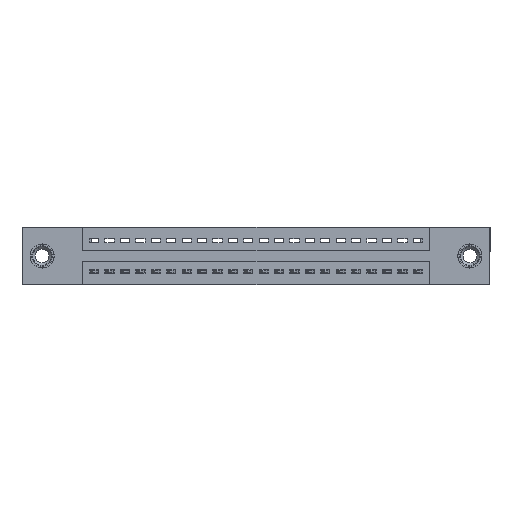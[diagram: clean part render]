
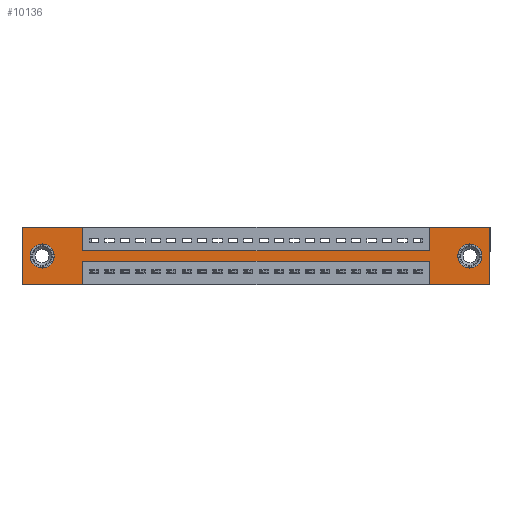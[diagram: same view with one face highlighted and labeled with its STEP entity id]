
A CAD part, front view. The second image highlights one B-rep face of the part: STEP entity #10136.
In plain terms, the highlighted planar face has unit normal (0, -1, 0).
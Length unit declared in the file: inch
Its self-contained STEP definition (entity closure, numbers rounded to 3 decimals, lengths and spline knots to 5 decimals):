
#239 = CARTESIAN_POINT ( 'NONE',  ( 3.035, 0., 0. ) ) ;
#268 = VERTEX_POINT ( 'NONE', #17367 ) ;
#348 = CARTESIAN_POINT ( 'NONE',  ( 2.905, 0., -0.107 ) ) ;
#859 = ORIENTED_EDGE ( 'NONE', *, *, #13881, .T. ) ;
#918 = LINE ( 'NONE', #5117, #19272 ) ;
#1190 = ORIENTED_EDGE ( 'NONE', *, *, #11688, .T. ) ;
#1259 = CARTESIAN_POINT ( 'NONE',  ( 3.035, 0., -0.37 ) ) ;
#1475 = VECTOR ( 'NONE', #5747, 39.37008 ) ;
#1801 = FACE_BOUND ( 'NONE', #2413, .T. ) ;
#2102 = VECTOR ( 'NONE', #16016, 39.37008 ) ;
#2111 = CARTESIAN_POINT ( 'NONE',  ( 0.13, 0., -0.185 ) ) ;
#2248 = EDGE_LOOP ( 'NONE', ( #1190, #8141 ) ) ;
#2413 = EDGE_LOOP ( 'NONE', ( #859, #3671 ) ) ;
#2635 = PLANE ( 'NONE',  #16412 ) ;
#2833 = LINE ( 'NONE', #17756, #11356 ) ;
#3108 = CARTESIAN_POINT ( 'NONE',  ( 2.6425, 0., -0.22 ) ) ;
#3216 = CARTESIAN_POINT ( 'NONE',  ( 2.6425, 0., -0.37 ) ) ;
#3261 = CARTESIAN_POINT ( 'NONE',  ( 0., 0., -0.37 ) ) ;
#3460 = CARTESIAN_POINT ( 'NONE',  ( 0.3925, 0., -0.37 ) ) ;
#3671 = ORIENTED_EDGE ( 'NONE', *, *, #16153, .T. ) ;
#3738 = VECTOR ( 'NONE', #13665, 39.37008 ) ;
#3745 = VERTEX_POINT ( 'NONE', #17710 ) ;
#3965 = EDGE_CURVE ( 'NONE', #14811, #12699, #20220, .T. ) ;
#4048 = CIRCLE ( 'NONE', #10600, 0.078 ) ;
#4083 = CARTESIAN_POINT ( 'NONE',  ( 0., 0., -0.37 ) ) ;
#4700 = DIRECTION ( 'NONE',  ( 0., 0., -1. ) ) ;
#4835 = ORIENTED_EDGE ( 'NONE', *, *, #10574, .F. ) ;
#5117 = CARTESIAN_POINT ( 'NONE',  ( 0., 0., 0. ) ) ;
#5172 = FACE_OUTER_BOUND ( 'NONE', #19229, .T. ) ;
#5348 = ORIENTED_EDGE ( 'NONE', *, *, #20519, .F. ) ;
#5518 = EDGE_CURVE ( 'NONE', #268, #15075, #14728, .T. ) ;
#5523 = AXIS2_PLACEMENT_3D ( 'NONE', #21179, #11009, #7885 ) ;
#5589 = DIRECTION ( 'NONE',  ( 0., 0., 1. ) ) ;
#5600 = CARTESIAN_POINT ( 'NONE',  ( 2.905, 0., -0.263 ) ) ;
#5620 = EDGE_CURVE ( 'NONE', #21409, #8973, #2833, .T. ) ;
#5747 = DIRECTION ( 'NONE',  ( 0., 0., -1. ) ) ;
#5774 = VERTEX_POINT ( 'NONE', #9091 ) ;
#5919 = FACE_BOUND ( 'NONE', #2248, .T. ) ;
#5966 = VECTOR ( 'NONE', #13341, 39.37008 ) ;
#6028 = VERTEX_POINT ( 'NONE', #9609 ) ;
#6134 = ORIENTED_EDGE ( 'NONE', *, *, #20076, .F. ) ;
#6158 = CARTESIAN_POINT ( 'NONE',  ( 0., 0., 0. ) ) ;
#6594 = EDGE_CURVE ( 'NONE', #7924, #11607, #6662, .T. ) ;
#6662 = LINE ( 'NONE', #12467, #17258 ) ;
#6959 = CARTESIAN_POINT ( 'NONE',  ( 0.13, 0., -0.185 ) ) ;
#7037 = CARTESIAN_POINT ( 'NONE',  ( 0.13, 0., -0.263 ) ) ;
#7156 = DIRECTION ( 'NONE',  ( 0., 0., -1. ) ) ;
#7234 = EDGE_CURVE ( 'NONE', #5774, #7924, #19030, .T. ) ;
#7763 = DIRECTION ( 'NONE',  ( 0., 0., 1. ) ) ;
#7828 = EDGE_CURVE ( 'NONE', #17112, #3745, #918, .T. ) ;
#7885 = DIRECTION ( 'NONE',  ( 0., 0., -1. ) ) ;
#7916 = CARTESIAN_POINT ( 'NONE',  ( 2.6425, 0., -0.15 ) ) ;
#7924 = VERTEX_POINT ( 'NONE', #9807 ) ;
#7933 = CARTESIAN_POINT ( 'NONE',  ( 2.905, 0., -0.185 ) ) ;
#8141 = ORIENTED_EDGE ( 'NONE', *, *, #3965, .T. ) ;
#8830 = DIRECTION ( 'NONE',  ( 0., 1., 0. ) ) ;
#8924 = LINE ( 'NONE', #6158, #18744 ) ;
#8973 = VERTEX_POINT ( 'NONE', #3108 ) ;
#9091 = CARTESIAN_POINT ( 'NONE',  ( 0.3925, 0., 0. ) ) ;
#9251 = DIRECTION ( 'NONE',  ( 1., 0., 0. ) ) ;
#9600 = LINE ( 'NONE', #16467, #14000 ) ;
#9609 = CARTESIAN_POINT ( 'NONE',  ( 2.6425, 0., 0. ) ) ;
#9770 = VECTOR ( 'NONE', #14161, 39.37008 ) ;
#9807 = CARTESIAN_POINT ( 'NONE',  ( 0.3925, 0., -0.15 ) ) ;
#10136 = ADVANCED_FACE ( 'NONE', ( #1801, #5919, #5172 ), #2635, .T. ) ;
#10286 = CIRCLE ( 'NONE', #14412, 0.078 ) ;
#10334 = VERTEX_POINT ( 'NONE', #348 ) ;
#10574 = EDGE_CURVE ( 'NONE', #8973, #268, #19335, .T. ) ;
#10600 = AXIS2_PLACEMENT_3D ( 'NONE', #2111, #8830, #5589 ) ;
#10656 = CARTESIAN_POINT ( 'NONE',  ( 0.3925, 0., 0. ) ) ;
#10718 = ORIENTED_EDGE ( 'NONE', *, *, #7828, .F. ) ;
#10991 = CARTESIAN_POINT ( 'NONE',  ( 0.3925, 0., -0.22 ) ) ;
#11009 = DIRECTION ( 'NONE',  ( 0., 1., 0. ) ) ;
#11266 = DIRECTION ( 'NONE',  ( 0., 1., 0. ) ) ;
#11284 = DIRECTION ( 'NONE',  ( 1., 0., 0. ) ) ;
#11356 = VECTOR ( 'NONE', #7763, 39.37008 ) ;
#11607 = VERTEX_POINT ( 'NONE', #7916 ) ;
#11688 = EDGE_CURVE ( 'NONE', #12699, #14811, #4048, .T. ) ;
#11885 = ORIENTED_EDGE ( 'NONE', *, *, #14466, .F. ) ;
#11907 = LINE ( 'NONE', #3261, #5966 ) ;
#12123 = DIRECTION ( 'NONE',  ( 0., 1., 0. ) ) ;
#12148 = LINE ( 'NONE', #12590, #2102 ) ;
#12467 = CARTESIAN_POINT ( 'NONE',  ( 0.3925, 0., -0.15 ) ) ;
#12487 = CARTESIAN_POINT ( 'NONE',  ( 0., 0., -0.37 ) ) ;
#12590 = CARTESIAN_POINT ( 'NONE',  ( 3.035, 0., 0. ) ) ;
#12699 = VERTEX_POINT ( 'NONE', #14220 ) ;
#12787 = ORIENTED_EDGE ( 'NONE', *, *, #5518, .F. ) ;
#13257 = LINE ( 'NONE', #12487, #19224 ) ;
#13325 = VERTEX_POINT ( 'NONE', #5600 ) ;
#13341 = DIRECTION ( 'NONE',  ( -1., 0., 0. ) ) ;
#13421 = DIRECTION ( 'NONE',  ( 0., 0., 1. ) ) ;
#13665 = DIRECTION ( 'NONE',  ( 1., 0., 0. ) ) ;
#13773 = ORIENTED_EDGE ( 'NONE', *, *, #18605, .F. ) ;
#13805 = LINE ( 'NONE', #19731, #3738 ) ;
#13881 = EDGE_CURVE ( 'NONE', #10334, #13325, #18911, .T. ) ;
#13932 = ORIENTED_EDGE ( 'NONE', *, *, #17863, .F. ) ;
#14000 = VECTOR ( 'NONE', #13421, 39.37008 ) ;
#14161 = DIRECTION ( 'NONE',  ( -1., 0., 0. ) ) ;
#14191 = DIRECTION ( 'NONE',  ( 0., 0., -1. ) ) ;
#14220 = CARTESIAN_POINT ( 'NONE',  ( 0.13, 0., -0.107 ) ) ;
#14412 = AXIS2_PLACEMENT_3D ( 'NONE', #7933, #11266, #4700 ) ;
#14466 = EDGE_CURVE ( 'NONE', #15075, #17112, #11907, .T. ) ;
#14728 = LINE ( 'NONE', #16998, #17053 ) ;
#14811 = VERTEX_POINT ( 'NONE', #7037 ) ;
#14993 = VERTEX_POINT ( 'NONE', #1259 ) ;
#15075 = VERTEX_POINT ( 'NONE', #3460 ) ;
#16016 = DIRECTION ( 'NONE',  ( 0., 0., -1. ) ) ;
#16028 = ORIENTED_EDGE ( 'NONE', *, *, #21431, .F. ) ;
#16153 = EDGE_CURVE ( 'NONE', #13325, #10334, #10286, .T. ) ;
#16412 = AXIS2_PLACEMENT_3D ( 'NONE', #4083, #20684, #14191 ) ;
#16467 = CARTESIAN_POINT ( 'NONE',  ( 2.6425, 0., 0. ) ) ;
#16543 = CARTESIAN_POINT ( 'NONE',  ( 0., 0., -0.37 ) ) ;
#16998 = CARTESIAN_POINT ( 'NONE',  ( 0.3925, 0., -0.37 ) ) ;
#17053 = VECTOR ( 'NONE', #7156, 39.37008 ) ;
#17112 = VERTEX_POINT ( 'NONE', #16543 ) ;
#17258 = VECTOR ( 'NONE', #9251, 39.37008 ) ;
#17367 = CARTESIAN_POINT ( 'NONE',  ( 0.3925, 0., -0.22 ) ) ;
#17710 = CARTESIAN_POINT ( 'NONE',  ( 0., 0., 0. ) ) ;
#17756 = CARTESIAN_POINT ( 'NONE',  ( 2.6425, 0., -0.37 ) ) ;
#17863 = EDGE_CURVE ( 'NONE', #3745, #5774, #8924, .T. ) ;
#18183 = DIRECTION ( 'NONE',  ( 0., 0., 1. ) ) ;
#18314 = ORIENTED_EDGE ( 'NONE', *, *, #5620, .F. ) ;
#18605 = EDGE_CURVE ( 'NONE', #14993, #21409, #13257, .T. ) ;
#18645 = DIRECTION ( 'NONE',  ( 0., 0., 1. ) ) ;
#18744 = VECTOR ( 'NONE', #11284, 39.37008 ) ;
#18911 = CIRCLE ( 'NONE', #5523, 0.078 ) ;
#19030 = LINE ( 'NONE', #10656, #1475 ) ;
#19062 = VERTEX_POINT ( 'NONE', #239 ) ;
#19079 = DIRECTION ( 'NONE',  ( -1., 0., 0. ) ) ;
#19224 = VECTOR ( 'NONE', #19079, 39.37008 ) ;
#19229 = EDGE_LOOP ( 'NONE', ( #12787, #4835, #18314, #13773, #5348, #16028, #6134, #20193, #19723, #13932, #10718, #11885 ) ) ;
#19272 = VECTOR ( 'NONE', #18183, 39.37008 ) ;
#19335 = LINE ( 'NONE', #10991, #9770 ) ;
#19723 = ORIENTED_EDGE ( 'NONE', *, *, #7234, .F. ) ;
#19731 = CARTESIAN_POINT ( 'NONE',  ( 0., 0., 0. ) ) ;
#19938 = AXIS2_PLACEMENT_3D ( 'NONE', #6959, #12123, #18645 ) ;
#20076 = EDGE_CURVE ( 'NONE', #11607, #6028, #9600, .T. ) ;
#20193 = ORIENTED_EDGE ( 'NONE', *, *, #6594, .F. ) ;
#20220 = CIRCLE ( 'NONE', #19938, 0.078 ) ;
#20519 = EDGE_CURVE ( 'NONE', #19062, #14993, #12148, .T. ) ;
#20684 = DIRECTION ( 'NONE',  ( 0., -1., 0. ) ) ;
#21179 = CARTESIAN_POINT ( 'NONE',  ( 2.905, 0., -0.185 ) ) ;
#21409 = VERTEX_POINT ( 'NONE', #3216 ) ;
#21431 = EDGE_CURVE ( 'NONE', #6028, #19062, #13805, .T. ) ;
